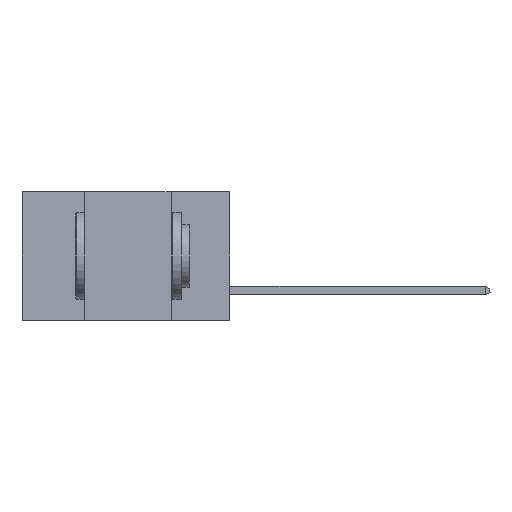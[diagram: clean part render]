
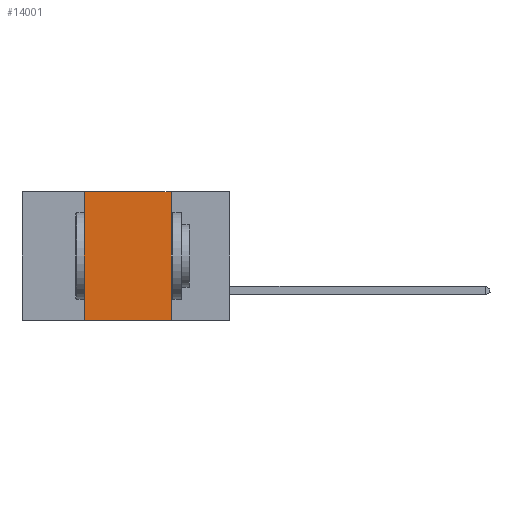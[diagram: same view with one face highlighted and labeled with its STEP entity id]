
A CAD part, left-side view. The second image highlights one B-rep face of the part: STEP entity #14001.
In plain terms, the highlighted planar face has unit normal (-1, 0, 0).
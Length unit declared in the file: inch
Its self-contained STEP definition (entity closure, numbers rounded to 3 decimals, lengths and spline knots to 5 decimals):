
#29 = AXIS2_PLACEMENT_3D ( 'NONE', #17579, #19722, #21834 ) ;
#281 = EDGE_CURVE ( 'NONE', #4923, #23535, #10333, .T. ) ;
#376 = FACE_OUTER_BOUND ( 'NONE', #19726, .T. ) ;
#3111 = DIRECTION ( 'NONE',  ( 0., 0., -1. ) ) ;
#4249 = VECTOR ( 'NONE', #14999, 39.37008 ) ;
#4539 = EDGE_CURVE ( 'NONE', #5676, #4923, #18964, .T. ) ;
#4923 = VERTEX_POINT ( 'NONE', #21173 ) ;
#5676 = VERTEX_POINT ( 'NONE', #7650 ) ;
#6581 = EDGE_CURVE ( 'NONE', #5676, #16738, #25809, .T. ) ;
#7650 = CARTESIAN_POINT ( 'NONE',  ( 0., 0.42, -0.37 ) ) ;
#7995 = VECTOR ( 'NONE', #3111, 39.37008 ) ;
#10314 = DIRECTION ( 'NONE',  ( 0., 0., 1. ) ) ;
#10333 = LINE ( 'NONE', #24778, #25270 ) ;
#11263 = PLANE ( 'NONE',  #29 ) ;
#12569 = ORIENTED_EDGE ( 'NONE', *, *, #281, .F. ) ;
#14001 = ADVANCED_FACE ( 'NONE', ( #376 ), #11263, .F. ) ;
#14473 = CARTESIAN_POINT ( 'NONE',  ( 0., 0.17, -0.37 ) ) ;
#14999 = DIRECTION ( 'NONE',  ( 0., -1., 0. ) ) ;
#16738 = VERTEX_POINT ( 'NONE', #14473 ) ;
#17579 = CARTESIAN_POINT ( 'NONE',  ( 0., 0.6, 0. ) ) ;
#18565 = EDGE_CURVE ( 'NONE', #23535, #16738, #24593, .T. ) ;
#18964 = LINE ( 'NONE', #20681, #21265 ) ;
#19722 = DIRECTION ( 'NONE',  ( 1., 0., 0. ) ) ;
#19726 = EDGE_LOOP ( 'NONE', ( #21297, #12569, #22952, #27445 ) ) ;
#20442 = CARTESIAN_POINT ( 'NONE',  ( 0., 0.17, 0. ) ) ;
#20681 = CARTESIAN_POINT ( 'NONE',  ( 0., 0.42, 0. ) ) ;
#21173 = CARTESIAN_POINT ( 'NONE',  ( 0., 0.42, 0. ) ) ;
#21265 = VECTOR ( 'NONE', #10314, 39.37008 ) ;
#21297 = ORIENTED_EDGE ( 'NONE', *, *, #18565, .F. ) ;
#21834 = DIRECTION ( 'NONE',  ( 0., 0., -1. ) ) ;
#22706 = DIRECTION ( 'NONE',  ( 0., -1., 0. ) ) ;
#22952 = ORIENTED_EDGE ( 'NONE', *, *, #4539, .F. ) ;
#23535 = VERTEX_POINT ( 'NONE', #20442 ) ;
#24593 = LINE ( 'NONE', #26222, #7995 ) ;
#24778 = CARTESIAN_POINT ( 'NONE',  ( 0., 0.6, 0. ) ) ;
#25270 = VECTOR ( 'NONE', #22706, 39.37008 ) ;
#25809 = LINE ( 'NONE', #25894, #4249 ) ;
#25894 = CARTESIAN_POINT ( 'NONE',  ( 0., 0.6, -0.37 ) ) ;
#26222 = CARTESIAN_POINT ( 'NONE',  ( 0., 0.17, 0. ) ) ;
#27445 = ORIENTED_EDGE ( 'NONE', *, *, #6581, .T. ) ;
